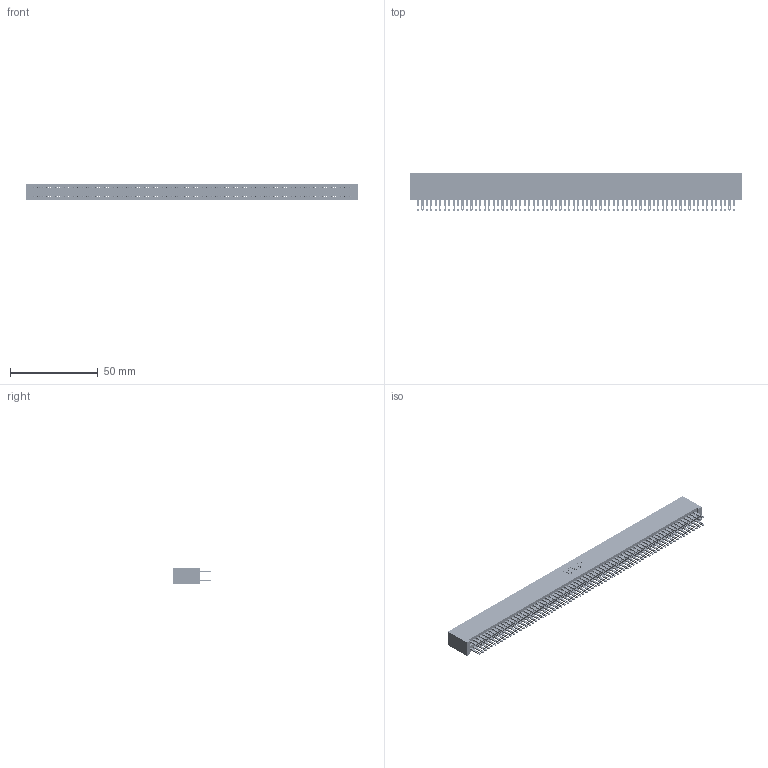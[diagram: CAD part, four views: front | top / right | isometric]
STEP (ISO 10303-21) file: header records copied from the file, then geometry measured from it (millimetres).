
FILE_DESCRIPTION (( 'STEP AP203' ), '1' );
FILE_NAME ('345-144-500-201.STEP', '2018-10-22T14:50:31', ( '' ), ( '' ), 'SwSTEP 2.0', 'SolidWorks 2016', '' );
FILE_SCHEMA (( 'CONFIG_CONTROL_DESIGN' ));
Length unit declared in the file: inch
Products named in the file (3): 345-144-500-201; 345-292-001_345-293-100; 345 Part_No Mounting Lugs
Assembly tree (145 placements, depth 2):
  345-144-500-201
    345 Part_No Mounting Lugs
    345-292-001_345-293-100  x144
Bounding box: 189.48 x 21.51 x 9.4 mm (x, y, z)
Volume: 19741.1 mm3; surface area: 31533.7 mm2
Topology: 145 solids, 145 shells, 6742 faces, 20621 edges, 13746 vertices
Faces by surface type: plane 3964, cylinder 2778
Entity records: 52107 total; most frequent: CARTESIAN_POINT 8704, ORIENTED_EDGE 8638, DIRECTION 7635, EDGE_CURVE 4319, VECTOR 3903, LINE 3903, VERTEX_POINT 2878, AXIS2_PLACEMENT_3D 1866
